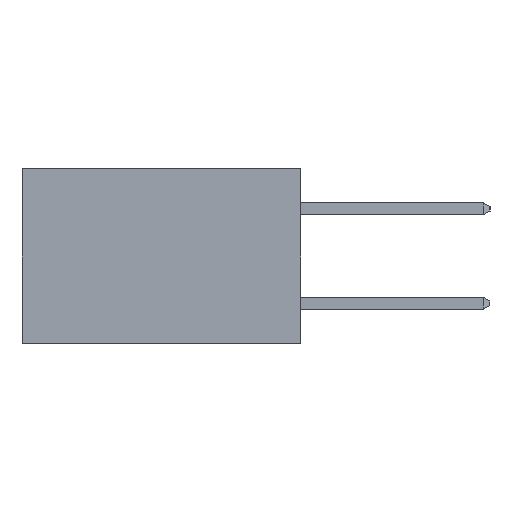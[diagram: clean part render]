
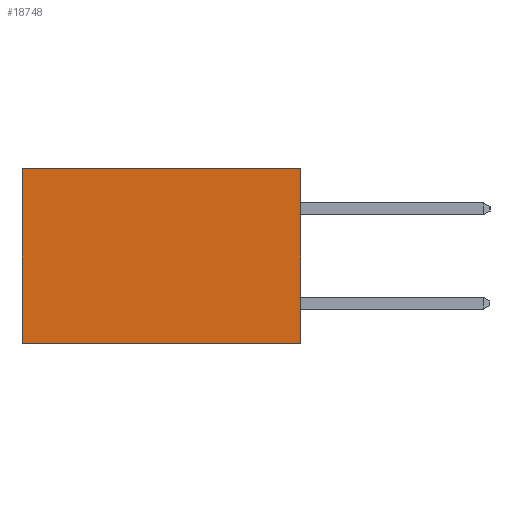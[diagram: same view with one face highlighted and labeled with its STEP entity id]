
A CAD part, left-side view. The second image highlights one B-rep face of the part: STEP entity #18748.
In plain terms, the highlighted planar face has unit normal (-1, 0, 0).
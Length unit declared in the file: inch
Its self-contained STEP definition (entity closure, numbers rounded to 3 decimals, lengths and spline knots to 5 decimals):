
#126 = VERTEX_POINT ( 'NONE', #11752 ) ;
#166 = DIRECTION ( 'NONE',  ( 0., 1., 0. ) ) ;
#212 = VECTOR ( 'NONE', #166, 39.37008 ) ;
#1929 = CARTESIAN_POINT ( 'NONE',  ( 0.277, 0., -0.37 ) ) ;
#2388 = CARTESIAN_POINT ( 'NONE',  ( 0.277, 0.59, -0.37 ) ) ;
#2940 = VERTEX_POINT ( 'NONE', #2388 ) ;
#3831 = DIRECTION ( 'NONE',  ( 0., 1., 0. ) ) ;
#4133 = DIRECTION ( 'NONE',  ( 0., 0., -1. ) ) ;
#5314 = ORIENTED_EDGE ( 'NONE', *, *, #9698, .F. ) ;
#5963 = VERTEX_POINT ( 'NONE', #24815 ) ;
#6436 = VECTOR ( 'NONE', #3831, 39.37008 ) ;
#7893 = CARTESIAN_POINT ( 'NONE',  ( 0.277, 0.59, -0.37 ) ) ;
#7897 = VECTOR ( 'NONE', #15728, 39.37008 ) ;
#8404 = VECTOR ( 'NONE', #18958, 39.37008 ) ;
#9474 = EDGE_CURVE ( 'NONE', #13295, #126, #24871, .T. ) ;
#9698 = EDGE_CURVE ( 'NONE', #5963, #2940, #23800, .T. ) ;
#10791 = PLANE ( 'NONE',  #18174 ) ;
#11235 = CARTESIAN_POINT ( 'NONE',  ( 0.277, 0., -0.37 ) ) ;
#11752 = CARTESIAN_POINT ( 'NONE',  ( 0.277, 0.59, 0. ) ) ;
#12726 = CARTESIAN_POINT ( 'NONE',  ( 0.277, 0., 0. ) ) ;
#13295 = VERTEX_POINT ( 'NONE', #21605 ) ;
#14669 = ORIENTED_EDGE ( 'NONE', *, *, #26703, .F. ) ;
#15728 = DIRECTION ( 'NONE',  ( 0., 0., -1. ) ) ;
#17461 = DIRECTION ( 'NONE',  ( 1., 0., 0. ) ) ;
#18174 = AXIS2_PLACEMENT_3D ( 'NONE', #1929, #17461, #4133 ) ;
#18748 = ADVANCED_FACE ( 'NONE', ( #20820 ), #10791, .F. ) ;
#18958 = DIRECTION ( 'NONE',  ( 0., 0., -1. ) ) ;
#19489 = LINE ( 'NONE', #7893, #8404 ) ;
#20082 = CARTESIAN_POINT ( 'NONE',  ( 0.277, 0., -0.37 ) ) ;
#20245 = EDGE_LOOP ( 'NONE', ( #28541, #5314, #14669, #21069 ) ) ;
#20820 = FACE_OUTER_BOUND ( 'NONE', #20245, .T. ) ;
#21069 = ORIENTED_EDGE ( 'NONE', *, *, #9474, .T. ) ;
#21605 = CARTESIAN_POINT ( 'NONE',  ( 0.277, 0., 0. ) ) ;
#23800 = LINE ( 'NONE', #11235, #212 ) ;
#24227 = EDGE_CURVE ( 'NONE', #126, #2940, #19489, .T. ) ;
#24815 = CARTESIAN_POINT ( 'NONE',  ( 0.277, 0., -0.37 ) ) ;
#24871 = LINE ( 'NONE', #12726, #6436 ) ;
#24922 = LINE ( 'NONE', #20082, #7897 ) ;
#26703 = EDGE_CURVE ( 'NONE', #13295, #5963, #24922, .T. ) ;
#28541 = ORIENTED_EDGE ( 'NONE', *, *, #24227, .T. ) ;
